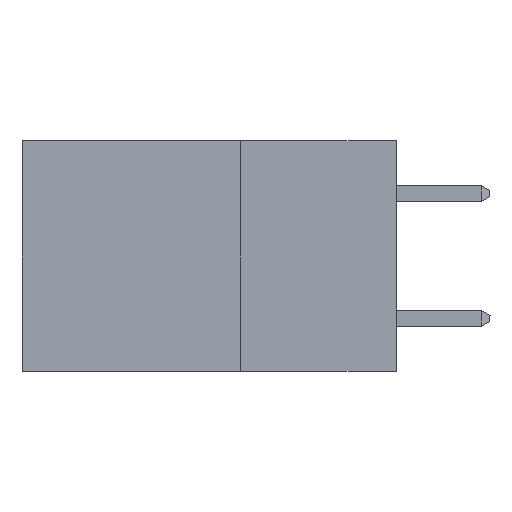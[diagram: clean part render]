
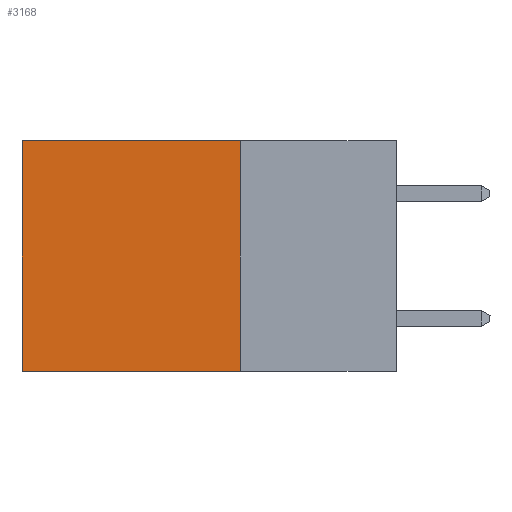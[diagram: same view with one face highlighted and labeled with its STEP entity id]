
A CAD part, left-side view. The second image highlights one B-rep face of the part: STEP entity #3168.
In plain terms, the highlighted planar face has unit normal (-1, 0, 0).
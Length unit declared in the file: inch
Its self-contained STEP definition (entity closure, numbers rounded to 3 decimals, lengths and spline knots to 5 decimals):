
#46 = EDGE_CURVE ( 'NONE', #10783, #5124, #2467, .T. ) ;
#997 = CARTESIAN_POINT ( 'NONE',  ( 0.2615, 0.25, -0.37 ) ) ;
#1058 = CARTESIAN_POINT ( 'NONE',  ( 0.2615, 0.25, -0.37 ) ) ;
#1289 = EDGE_LOOP ( 'NONE', ( #5425, #8136, #13776, #9166 ) ) ;
#1447 = VECTOR ( 'NONE', #4820, 39.37008 ) ;
#2467 = LINE ( 'NONE', #6576, #4971 ) ;
#2617 = CARTESIAN_POINT ( 'NONE',  ( 0.2615, 0.6, 0. ) ) ;
#3168 = ADVANCED_FACE ( 'NONE', ( #6132 ), #9466, .F. ) ;
#3617 = DIRECTION ( 'NONE',  ( 0., 0., -1. ) ) ;
#4328 = LINE ( 'NONE', #1058, #1447 ) ;
#4820 = DIRECTION ( 'NONE',  ( 0., 1., 0. ) ) ;
#4971 = VECTOR ( 'NONE', #8755, 39.37008 ) ;
#4985 = VECTOR ( 'NONE', #13190, 39.37008 ) ;
#5124 = VERTEX_POINT ( 'NONE', #2617 ) ;
#5329 = VECTOR ( 'NONE', #3617, 39.37008 ) ;
#5425 = ORIENTED_EDGE ( 'NONE', *, *, #7780, .T. ) ;
#5680 = LINE ( 'NONE', #10296, #5329 ) ;
#6132 = FACE_OUTER_BOUND ( 'NONE', #1289, .T. ) ;
#6576 = CARTESIAN_POINT ( 'NONE',  ( 0.2615, 0.25, 0. ) ) ;
#7280 = EDGE_CURVE ( 'NONE', #7364, #9754, #4328, .T. ) ;
#7364 = VERTEX_POINT ( 'NONE', #997 ) ;
#7780 = EDGE_CURVE ( 'NONE', #5124, #9754, #10254, .T. ) ;
#8136 = ORIENTED_EDGE ( 'NONE', *, *, #7280, .F. ) ;
#8755 = DIRECTION ( 'NONE',  ( 0., 1., 0. ) ) ;
#8756 = AXIS2_PLACEMENT_3D ( 'NONE', #9356, #9205, #9185 ) ;
#9166 = ORIENTED_EDGE ( 'NONE', *, *, #46, .T. ) ;
#9185 = DIRECTION ( 'NONE',  ( 0., 0., -1. ) ) ;
#9205 = DIRECTION ( 'NONE',  ( 1., 0., 0. ) ) ;
#9356 = CARTESIAN_POINT ( 'NONE',  ( 0.2615, 0.25, -0.37 ) ) ;
#9466 = PLANE ( 'NONE',  #8756 ) ;
#9754 = VERTEX_POINT ( 'NONE', #12309 ) ;
#10254 = LINE ( 'NONE', #13820, #4985 ) ;
#10296 = CARTESIAN_POINT ( 'NONE',  ( 0.2615, 0.25, -0.37 ) ) ;
#10783 = VERTEX_POINT ( 'NONE', #13889 ) ;
#12309 = CARTESIAN_POINT ( 'NONE',  ( 0.2615, 0.6, -0.37 ) ) ;
#13190 = DIRECTION ( 'NONE',  ( 0., 0., -1. ) ) ;
#13370 = EDGE_CURVE ( 'NONE', #10783, #7364, #5680, .T. ) ;
#13776 = ORIENTED_EDGE ( 'NONE', *, *, #13370, .F. ) ;
#13820 = CARTESIAN_POINT ( 'NONE',  ( 0.2615, 0.6, -0.37 ) ) ;
#13889 = CARTESIAN_POINT ( 'NONE',  ( 0.2615, 0.25, 0. ) ) ;
